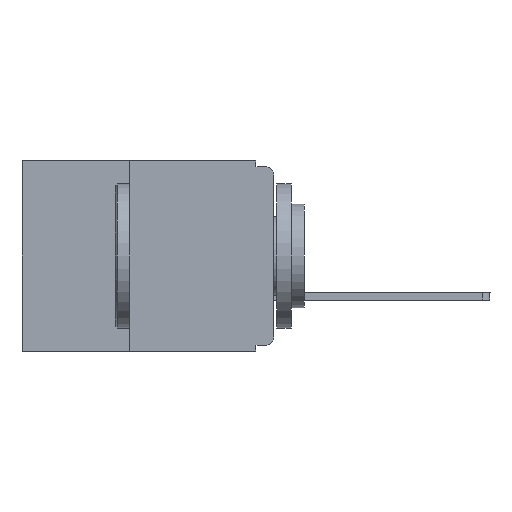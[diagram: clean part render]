
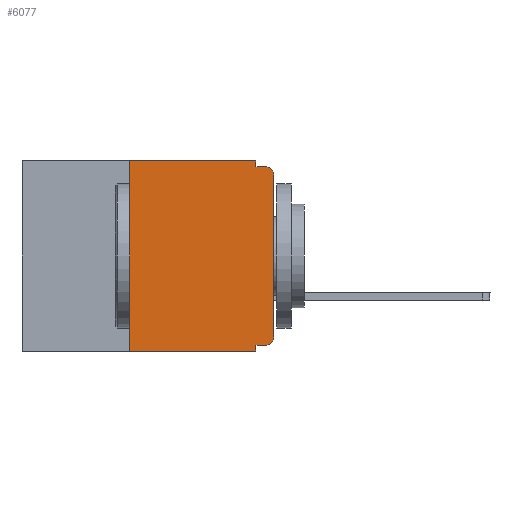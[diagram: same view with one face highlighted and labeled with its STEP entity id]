
A CAD part, left-side view. The second image highlights one B-rep face of the part: STEP entity #6077.
In plain terms, the highlighted planar face has unit normal (-1, 0, 0).
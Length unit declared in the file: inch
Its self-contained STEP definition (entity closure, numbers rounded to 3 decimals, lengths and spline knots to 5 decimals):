
#221 = CARTESIAN_POINT ( 'NONE',  ( 0., 0.25, -0.33 ) ) ;
#321 = VECTOR ( 'NONE', #11705, 39.37008 ) ;
#595 = VERTEX_POINT ( 'NONE', #3238 ) ;
#636 = VECTOR ( 'NONE', #5826, 39.37008 ) ;
#724 = DIRECTION ( 'NONE',  ( 0., 1., 0. ) ) ;
#745 = CARTESIAN_POINT ( 'NONE',  ( 0., 0.015, -0.305 ) ) ;
#838 = EDGE_CURVE ( 'NONE', #595, #4464, #3339, .T. ) ;
#1023 = DIRECTION ( 'NONE',  ( 1., 0., 0. ) ) ;
#1101 = VERTEX_POINT ( 'NONE', #4058 ) ;
#1234 = EDGE_CURVE ( 'NONE', #4516, #11053, #10529, .T. ) ;
#1742 = DIRECTION ( 'NONE',  ( -1., 0., 0. ) ) ;
#1746 = FACE_OUTER_BOUND ( 'NONE', #9645, .T. ) ;
#1773 = VERTEX_POINT ( 'NONE', #12298 ) ;
#1939 = CARTESIAN_POINT ( 'NONE',  ( 0., 0.031, -0.33 ) ) ;
#2028 = PLANE ( 'NONE',  #3301 ) ;
#2205 = ORIENTED_EDGE ( 'NONE', *, *, #6841, .T. ) ;
#2271 = AXIS2_PLACEMENT_3D ( 'NONE', #745, #1742, #8732 ) ;
#2660 = VECTOR ( 'NONE', #5493, 39.37008 ) ;
#2749 = EDGE_CURVE ( 'NONE', #4516, #10358, #9504, .T. ) ;
#2899 = CARTESIAN_POINT ( 'NONE',  ( 0., 0.25, 0. ) ) ;
#3112 = CARTESIAN_POINT ( 'NONE',  ( 0., 0.031, -0.33 ) ) ;
#3116 = ORIENTED_EDGE ( 'NONE', *, *, #5610, .T. ) ;
#3238 = CARTESIAN_POINT ( 'NONE',  ( 0., 0.015, -0.32 ) ) ;
#3301 = AXIS2_PLACEMENT_3D ( 'NONE', #8972, #1023, #8074 ) ;
#3339 = LINE ( 'NONE', #3611, #3781 ) ;
#3611 = CARTESIAN_POINT ( 'NONE',  ( 0., 0., -0.32 ) ) ;
#3781 = VECTOR ( 'NONE', #724, 39.37008 ) ;
#4044 = EDGE_CURVE ( 'NONE', #4464, #10358, #10398, .T. ) ;
#4058 = CARTESIAN_POINT ( 'NONE',  ( 0., 0., -0.025 ) ) ;
#4223 = VECTOR ( 'NONE', #12317, 39.37008 ) ;
#4349 = ORIENTED_EDGE ( 'NONE', *, *, #6773, .F. ) ;
#4464 = VERTEX_POINT ( 'NONE', #8045 ) ;
#4516 = VERTEX_POINT ( 'NONE', #221 ) ;
#4590 = ORIENTED_EDGE ( 'NONE', *, *, #6300, .F. ) ;
#4617 = DIRECTION ( 'NONE',  ( 0., 0., -1. ) ) ;
#4751 = VERTEX_POINT ( 'NONE', #8249 ) ;
#5331 = AXIS2_PLACEMENT_3D ( 'NONE', #11149, #9137, #12193 ) ;
#5351 = ORIENTED_EDGE ( 'NONE', *, *, #4044, .F. ) ;
#5397 = VECTOR ( 'NONE', #4617, 39.37008 ) ;
#5493 = DIRECTION ( 'NONE',  ( 0., -1., 0. ) ) ;
#5542 = CARTESIAN_POINT ( 'NONE',  ( 0., 0., -0.01 ) ) ;
#5587 = CIRCLE ( 'NONE', #5331, 0.015 ) ;
#5610 = EDGE_CURVE ( 'NONE', #1101, #1773, #5587, .T. ) ;
#5613 = VERTEX_POINT ( 'NONE', #9097 ) ;
#5646 = CARTESIAN_POINT ( 'NONE',  ( 0., 0.437, 0. ) ) ;
#5674 = VECTOR ( 'NONE', #7969, 39.37008 ) ;
#5826 = DIRECTION ( 'NONE',  ( 0., 0., 1. ) ) ;
#5853 = LINE ( 'NONE', #5646, #321 ) ;
#6045 = LINE ( 'NONE', #7539, #5397 ) ;
#6077 = ADVANCED_FACE ( 'NONE', ( #1746 ), #2028, .F. ) ;
#6114 = VECTOR ( 'NONE', #11855, 39.37008 ) ;
#6300 = EDGE_CURVE ( 'NONE', #4751, #1773, #12665, .T. ) ;
#6773 = EDGE_CURVE ( 'NONE', #5613, #4751, #6045, .T. ) ;
#6841 = EDGE_CURVE ( 'NONE', #10801, #1101, #8767, .T. ) ;
#6979 = ORIENTED_EDGE ( 'NONE', *, *, #1234, .F. ) ;
#7303 = EDGE_CURVE ( 'NONE', #11053, #5613, #5853, .T. ) ;
#7539 = CARTESIAN_POINT ( 'NONE',  ( 0., 0.031, 0. ) ) ;
#7969 = DIRECTION ( 'NONE',  ( 0., -1., 0. ) ) ;
#8045 = CARTESIAN_POINT ( 'NONE',  ( 0., 0.031, -0.32 ) ) ;
#8074 = DIRECTION ( 'NONE',  ( 0., 0., -1. ) ) ;
#8249 = CARTESIAN_POINT ( 'NONE',  ( 0., 0.031, -0.01 ) ) ;
#8580 = ORIENTED_EDGE ( 'NONE', *, *, #2749, .T. ) ;
#8732 = DIRECTION ( 'NONE',  ( 0., 0., -1. ) ) ;
#8767 = LINE ( 'NONE', #10043, #636 ) ;
#8799 = ORIENTED_EDGE ( 'NONE', *, *, #10096, .T. ) ;
#8972 = CARTESIAN_POINT ( 'NONE',  ( 0., 0.437, 0. ) ) ;
#9048 = CARTESIAN_POINT ( 'NONE',  ( 0., 0.437, -0.33 ) ) ;
#9097 = CARTESIAN_POINT ( 'NONE',  ( 0., 0.031, 0. ) ) ;
#9137 = DIRECTION ( 'NONE',  ( -1., 0., 0. ) ) ;
#9190 = CARTESIAN_POINT ( 'NONE',  ( 0., 0.25, -0.33 ) ) ;
#9504 = LINE ( 'NONE', #9048, #5674 ) ;
#9645 = EDGE_LOOP ( 'NONE', ( #2205, #3116, #4590, #4349, #10968, #6979, #8580, #5351, #12927, #8799 ) ) ;
#10043 = CARTESIAN_POINT ( 'NONE',  ( 0., 0., 0. ) ) ;
#10096 = EDGE_CURVE ( 'NONE', #595, #10801, #11254, .T. ) ;
#10358 = VERTEX_POINT ( 'NONE', #3112 ) ;
#10398 = LINE ( 'NONE', #1939, #6114 ) ;
#10529 = LINE ( 'NONE', #9190, #4223 ) ;
#10801 = VERTEX_POINT ( 'NONE', #12392 ) ;
#10968 = ORIENTED_EDGE ( 'NONE', *, *, #7303, .F. ) ;
#11053 = VERTEX_POINT ( 'NONE', #2899 ) ;
#11149 = CARTESIAN_POINT ( 'NONE',  ( 0., 0.015, -0.025 ) ) ;
#11254 = CIRCLE ( 'NONE', #2271, 0.015 ) ;
#11705 = DIRECTION ( 'NONE',  ( 0., -1., 0. ) ) ;
#11855 = DIRECTION ( 'NONE',  ( 0., 0., -1. ) ) ;
#12193 = DIRECTION ( 'NONE',  ( 0., 0., -1. ) ) ;
#12298 = CARTESIAN_POINT ( 'NONE',  ( 0., 0.015, -0.01 ) ) ;
#12317 = DIRECTION ( 'NONE',  ( 0., 0., 1. ) ) ;
#12392 = CARTESIAN_POINT ( 'NONE',  ( 0., 0., -0.305 ) ) ;
#12665 = LINE ( 'NONE', #5542, #2660 ) ;
#12927 = ORIENTED_EDGE ( 'NONE', *, *, #838, .F. ) ;
